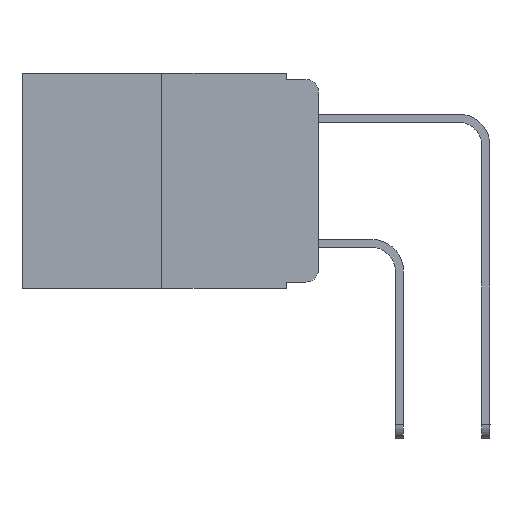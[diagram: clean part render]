
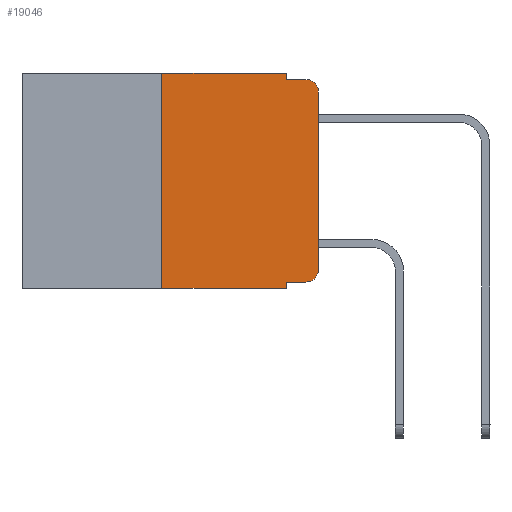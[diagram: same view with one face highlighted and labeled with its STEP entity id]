
A CAD part, left-side view. The second image highlights one B-rep face of the part: STEP entity #19046.
In plain terms, the highlighted planar face has unit normal (-1, 0, 0).
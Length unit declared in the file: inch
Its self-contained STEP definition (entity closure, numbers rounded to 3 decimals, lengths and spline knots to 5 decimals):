
#198 = DIRECTION ( 'NONE',  ( 0., 0., -1. ) ) ;
#417 = CARTESIAN_POINT ( 'NONE',  ( 0., 0.02, -0.01 ) ) ;
#1245 = ORIENTED_EDGE ( 'NONE', *, *, #2967, .T. ) ;
#1471 = VECTOR ( 'NONE', #13497, 39.37008 ) ;
#1736 = LINE ( 'NONE', #2155, #20476 ) ;
#1948 = CARTESIAN_POINT ( 'NONE',  ( 0., 0.051, 0. ) ) ;
#2048 = VERTEX_POINT ( 'NONE', #21824 ) ;
#2152 = VERTEX_POINT ( 'NONE', #16190 ) ;
#2155 = CARTESIAN_POINT ( 'NONE',  ( 0., 0., 0. ) ) ;
#2203 = CIRCLE ( 'NONE', #26608, 0.02 ) ;
#2813 = VERTEX_POINT ( 'NONE', #12530 ) ;
#2904 = VERTEX_POINT ( 'NONE', #14977 ) ;
#2967 = EDGE_CURVE ( 'NONE', #21516, #2813, #5415, .T. ) ;
#3012 = ORIENTED_EDGE ( 'NONE', *, *, #8623, .F. ) ;
#3042 = CARTESIAN_POINT ( 'NONE',  ( 0., 0.25, 0. ) ) ;
#3305 = DIRECTION ( 'NONE',  ( -1., 0., 0. ) ) ;
#3653 = VERTEX_POINT ( 'NONE', #8259 ) ;
#3679 = AXIS2_PLACEMENT_3D ( 'NONE', #16911, #25700, #23558 ) ;
#3904 = CARTESIAN_POINT ( 'NONE',  ( 0., 0.051, -0.333 ) ) ;
#4153 = EDGE_CURVE ( 'NONE', #26250, #3653, #24154, .T. ) ;
#4223 = VERTEX_POINT ( 'NONE', #24210 ) ;
#4263 = LINE ( 'NONE', #1948, #27360 ) ;
#4315 = CARTESIAN_POINT ( 'NONE',  ( 0., 0.02, -0.313 ) ) ;
#4714 = ORIENTED_EDGE ( 'NONE', *, *, #5079, .F. ) ;
#5001 = DIRECTION ( 'NONE',  ( 0., -1., 0. ) ) ;
#5079 = EDGE_CURVE ( 'NONE', #4223, #2813, #4263, .T. ) ;
#5415 = LINE ( 'NONE', #15950, #19934 ) ;
#5760 = AXIS2_PLACEMENT_3D ( 'NONE', #4315, #13240, #28253 ) ;
#6551 = CARTESIAN_POINT ( 'NONE',  ( 0., 0.473, 0. ) ) ;
#7810 = VECTOR ( 'NONE', #13710, 39.37008 ) ;
#7890 = ORIENTED_EDGE ( 'NONE', *, *, #4153, .T. ) ;
#8259 = CARTESIAN_POINT ( 'NONE',  ( 0., 0., -0.313 ) ) ;
#8623 = EDGE_CURVE ( 'NONE', #21516, #2152, #22794, .T. ) ;
#8831 = CARTESIAN_POINT ( 'NONE',  ( 0., 0.25, -0.343 ) ) ;
#9319 = VECTOR ( 'NONE', #10586, 39.37008 ) ;
#9475 = LINE ( 'NONE', #16096, #1471 ) ;
#10279 = PLANE ( 'NONE',  #3679 ) ;
#10311 = CARTESIAN_POINT ( 'NONE',  ( 0., 0.051, -0.01 ) ) ;
#10586 = DIRECTION ( 'NONE',  ( 0., -1., 0. ) ) ;
#10668 = LINE ( 'NONE', #3904, #12158 ) ;
#11574 = ORIENTED_EDGE ( 'NONE', *, *, #25489, .T. ) ;
#11958 = DIRECTION ( 'NONE',  ( 0., 0., -1. ) ) ;
#12158 = VECTOR ( 'NONE', #19460, 39.37008 ) ;
#12250 = EDGE_CURVE ( 'NONE', #2048, #25587, #2203, .T. ) ;
#12413 = CARTESIAN_POINT ( 'NONE',  ( 0., 0.051, 0. ) ) ;
#12530 = CARTESIAN_POINT ( 'NONE',  ( 0., 0.051, -0.343 ) ) ;
#13240 = DIRECTION ( 'NONE',  ( -1., 0., 0. ) ) ;
#13497 = DIRECTION ( 'NONE',  ( 0., -1., 0. ) ) ;
#13710 = DIRECTION ( 'NONE',  ( 0., 0., 1. ) ) ;
#14977 = CARTESIAN_POINT ( 'NONE',  ( 0., 0.051, 0. ) ) ;
#15950 = CARTESIAN_POINT ( 'NONE',  ( 0., 0.473, -0.343 ) ) ;
#16096 = CARTESIAN_POINT ( 'NONE',  ( 0., 0.051, -0.01 ) ) ;
#16190 = CARTESIAN_POINT ( 'NONE',  ( 0., 0.25, 0. ) ) ;
#16911 = CARTESIAN_POINT ( 'NONE',  ( 0., 0.473, 0. ) ) ;
#17392 = ORIENTED_EDGE ( 'NONE', *, *, #12250, .T. ) ;
#18436 = VERTEX_POINT ( 'NONE', #10311 ) ;
#19046 = ADVANCED_FACE ( 'NONE', ( #23412 ), #10279, .F. ) ;
#19323 = DIRECTION ( 'NONE',  ( 0., 0., -1. ) ) ;
#19460 = DIRECTION ( 'NONE',  ( 0., -1., 0. ) ) ;
#19523 = LINE ( 'NONE', #6551, #9319 ) ;
#19706 = ORIENTED_EDGE ( 'NONE', *, *, #27504, .F. ) ;
#19934 = VECTOR ( 'NONE', #5001, 39.37008 ) ;
#20025 = VECTOR ( 'NONE', #19323, 39.37008 ) ;
#20476 = VECTOR ( 'NONE', #21777, 39.37008 ) ;
#21500 = LINE ( 'NONE', #12413, #20025 ) ;
#21516 = VERTEX_POINT ( 'NONE', #8831 ) ;
#21777 = DIRECTION ( 'NONE',  ( 0., 0., 1. ) ) ;
#21824 = CARTESIAN_POINT ( 'NONE',  ( 0., 0., -0.03 ) ) ;
#22794 = LINE ( 'NONE', #3042, #7810 ) ;
#22906 = ORIENTED_EDGE ( 'NONE', *, *, #23331, .F. ) ;
#23021 = EDGE_CURVE ( 'NONE', #18436, #25587, #9475, .T. ) ;
#23331 = EDGE_CURVE ( 'NONE', #2152, #2904, #19523, .T. ) ;
#23412 = FACE_OUTER_BOUND ( 'NONE', #25053, .T. ) ;
#23558 = DIRECTION ( 'NONE',  ( 0., 0., -1. ) ) ;
#24154 = CIRCLE ( 'NONE', #5760, 0.02 ) ;
#24210 = CARTESIAN_POINT ( 'NONE',  ( 0., 0.051, -0.333 ) ) ;
#25053 = EDGE_LOOP ( 'NONE', ( #11574, #17392, #25480, #19706, #22906, #3012, #1245, #4714, #27931, #7890 ) ) ;
#25424 = EDGE_CURVE ( 'NONE', #4223, #26250, #10668, .T. ) ;
#25480 = ORIENTED_EDGE ( 'NONE', *, *, #23021, .F. ) ;
#25489 = EDGE_CURVE ( 'NONE', #3653, #2048, #1736, .T. ) ;
#25587 = VERTEX_POINT ( 'NONE', #417 ) ;
#25700 = DIRECTION ( 'NONE',  ( 1., 0., 0. ) ) ;
#25946 = CARTESIAN_POINT ( 'NONE',  ( 0., 0.02, -0.333 ) ) ;
#26250 = VERTEX_POINT ( 'NONE', #25946 ) ;
#26608 = AXIS2_PLACEMENT_3D ( 'NONE', #26957, #3305, #11958 ) ;
#26957 = CARTESIAN_POINT ( 'NONE',  ( 0., 0.02, -0.03 ) ) ;
#27360 = VECTOR ( 'NONE', #198, 39.37008 ) ;
#27504 = EDGE_CURVE ( 'NONE', #2904, #18436, #21500, .T. ) ;
#27931 = ORIENTED_EDGE ( 'NONE', *, *, #25424, .T. ) ;
#28253 = DIRECTION ( 'NONE',  ( 0., 0., -1. ) ) ;
